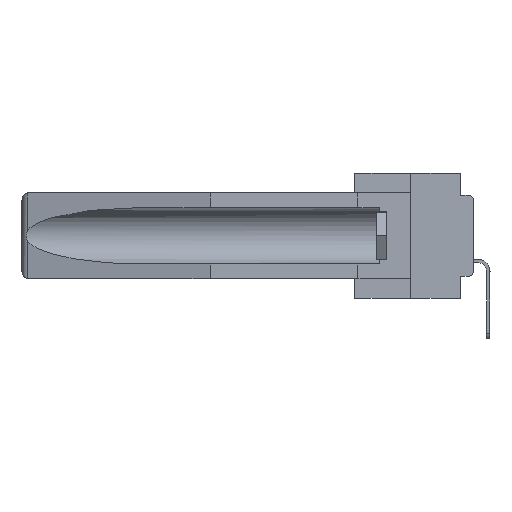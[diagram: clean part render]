
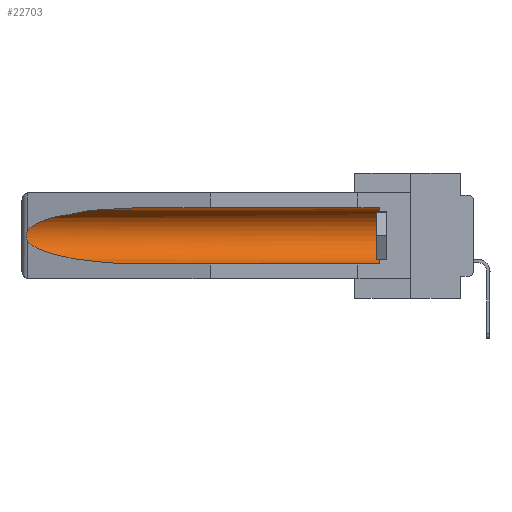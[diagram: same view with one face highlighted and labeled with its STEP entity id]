
A CAD part, left-side view. The second image highlights one B-rep face of the part: STEP entity #22703.
In plain terms, the highlighted cylindrical face has radius 2.857 mm (diameter 5.715 mm), a partial arc.
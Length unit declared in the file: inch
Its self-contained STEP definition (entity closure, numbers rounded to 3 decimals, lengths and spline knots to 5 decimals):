
#1661 = ORIENTED_EDGE ( 'NONE', *, *, #19579, .T. ) ;
#3295 = CARTESIAN_POINT ( 'NONE',  ( 0.2673, 1.5327, -0.16383 ) ) ;
#3520 = CARTESIAN_POINT ( 'NONE',  ( 0.155, 0.126, -0.059 ) ) ;
#3629 = EDGE_CURVE ( 'NONE', #25369, #14573, #30500, .T. ) ;
#4773 = EDGE_LOOP ( 'NONE', ( #11918, #1661, #10795, #9263, #9415, #20412 ) ) ;
#5623 = CARTESIAN_POINT ( 'NONE',  ( 0.26654, 1.53092, -0.15636 ) ) ;
#5877 = VECTOR ( 'NONE', #8339, 39.37008 ) ;
#6345 =( BOUNDED_CURVE ( )  B_SPLINE_CURVE ( 3, ( #18816, #21116, #14318, #19122 ),
 .UNSPECIFIED., .F., .F. ) 
 B_SPLINE_CURVE_WITH_KNOTS ( ( 4, 4 ),
 ( 0.1948, 1.5708 ),
 .UNSPECIFIED. ) 
 CURVE ( )  GEOMETRIC_REPRESENTATION_ITEM ( )  RATIONAL_B_SPLINE_CURVE ( ( 1., 0.848, 0.848, 1. ) ) 
 REPRESENTATION_ITEM ( '' )  );
#6880 = CARTESIAN_POINT ( 'NONE',  ( 0.26537, 1.52718, -0.19328 ) ) ;
#7287 = CARTESIAN_POINT ( 'NONE',  ( 0.155, 0.126, -0.1715 ) ) ;
#7567 = CARTESIAN_POINT ( 'NONE',  ( 0.155, 1.07973, -0.284 ) ) ;
#7580 = EDGE_CURVE ( 'NONE', #14573, #22712, #9837, .T. ) ;
#7781 = CARTESIAN_POINT ( 'NONE',  ( 0.2675, 1.53308, -0.17534 ) ) ;
#7938 = CARTESIAN_POINT ( 'NONE',  ( 0.26655, 1.53094, -0.18657 ) ) ;
#8052 = LINE ( 'NONE', #10712, #19145 ) ;
#8318 = CARTESIAN_POINT ( 'NONE',  ( 0.21114, 1.30732, -0.059 ) ) ;
#8339 = DIRECTION ( 'NONE',  ( 0., 1., 0. ) ) ;
#8440 = CARTESIAN_POINT ( 'NONE',  ( 0.26597, 1.52961, -0.15275 ) ) ;
#8776 = FACE_OUTER_BOUND ( 'NONE', #4773, .T. ) ;
#9240 = AXIS2_PLACEMENT_3D ( 'NONE', #21017, #23801, #31074 ) ;
#9263 = ORIENTED_EDGE ( 'NONE', *, *, #13579, .F. ) ;
#9415 = ORIENTED_EDGE ( 'NONE', *, *, #3629, .T. ) ;
#9731 =( BOUNDED_CURVE ( )  B_SPLINE_CURVE ( 3, ( #15768, #8318, #21047, #15606 ),
 .UNSPECIFIED., .F., .F. ) 
 B_SPLINE_CURVE_WITH_KNOTS ( ( 4, 4 ),
 ( 4.71239, 6.08839 ),
 .UNSPECIFIED. ) 
 CURVE ( )  GEOMETRIC_REPRESENTATION_ITEM ( )  RATIONAL_B_SPLINE_CURVE ( ( 1., 0.848, 0.848, 1. ) ) 
 REPRESENTATION_ITEM ( '' )  );
#9837 = LINE ( 'NONE', #19929, #5877 ) ;
#10291 = EDGE_CURVE ( 'NONE', #24259, #24067, #6345, .T. ) ;
#10712 = CARTESIAN_POINT ( 'NONE',  ( 0.155, -0.30754, -0.284 ) ) ;
#10795 = ORIENTED_EDGE ( 'NONE', *, *, #10291, .T. ) ;
#11918 = ORIENTED_EDGE ( 'NONE', *, *, #19132, .T. ) ;
#13579 = EDGE_CURVE ( 'NONE', #25369, #24067, #8052, .T. ) ;
#14318 = CARTESIAN_POINT ( 'NONE',  ( 0.21114, 1.30732, -0.284 ) ) ;
#14573 = VERTEX_POINT ( 'NONE', #3520 ) ;
#14882 = DIRECTION ( 'NONE',  ( 0., 0., 1. ) ) ;
#15201 = DIRECTION ( 'NONE',  ( 0., 1., 0. ) ) ;
#15606 = CARTESIAN_POINT ( 'NONE',  ( 0.26537, 1.52718, -0.14972 ) ) ;
#15768 = CARTESIAN_POINT ( 'NONE',  ( 0.155, 1.07973, -0.059 ) ) ;
#18533 = CARTESIAN_POINT ( 'NONE',  ( 0.2673, 1.53269, -0.17917 ) ) ;
#18542 = CARTESIAN_POINT ( 'NONE',  ( 0.155, 1.07973, -0.059 ) ) ;
#18816 = CARTESIAN_POINT ( 'NONE',  ( 0.26537, 1.52718, -0.19328 ) ) ;
#18875 = CYLINDRICAL_SURFACE ( 'NONE', #9240, 0.1125 ) ;
#19122 = CARTESIAN_POINT ( 'NONE',  ( 0.155, 1.07973, -0.284 ) ) ;
#19132 = EDGE_CURVE ( 'NONE', #22712, #27759, #9731, .T. ) ;
#19145 = VECTOR ( 'NONE', #15201, 39.37008 ) ;
#19579 = EDGE_CURVE ( 'NONE', #27759, #24259, #31575, .T. ) ;
#19929 = CARTESIAN_POINT ( 'NONE',  ( 0.155, -0.30754, -0.059 ) ) ;
#20354 = CARTESIAN_POINT ( 'NONE',  ( 0.26597, 1.5296, -0.19026 ) ) ;
#20412 = ORIENTED_EDGE ( 'NONE', *, *, #7580, .T. ) ;
#21017 = CARTESIAN_POINT ( 'NONE',  ( 0.155, -0.30754, -0.1715 ) ) ;
#21047 = CARTESIAN_POINT ( 'NONE',  ( 0.25451, 1.48313, -0.09465 ) ) ;
#21116 = CARTESIAN_POINT ( 'NONE',  ( 0.25451, 1.48313, -0.24835 ) ) ;
#22703 = ADVANCED_FACE ( 'NONE', ( #8776 ), #18875, .F. ) ;
#22712 = VERTEX_POINT ( 'NONE', #18542 ) ;
#22792 = DIRECTION ( 'NONE',  ( 0., -1., 0. ) ) ;
#23801 = DIRECTION ( 'NONE',  ( 0., 1., 0. ) ) ;
#24067 = VERTEX_POINT ( 'NONE', #7567 ) ;
#24259 = VERTEX_POINT ( 'NONE', #6880 ) ;
#25369 = VERTEX_POINT ( 'NONE', #28227 ) ;
#25634 = CARTESIAN_POINT ( 'NONE',  ( 0.26537, 1.52718, -0.14972 ) ) ;
#25984 = CARTESIAN_POINT ( 'NONE',  ( 0.26537, 1.52718, -0.14972 ) ) ;
#27328 = AXIS2_PLACEMENT_3D ( 'NONE', #7287, #22792, #14882 ) ;
#27759 = VERTEX_POINT ( 'NONE', #25984 ) ;
#28227 = CARTESIAN_POINT ( 'NONE',  ( 0.155, 0.126, -0.284 ) ) ;
#28586 = CARTESIAN_POINT ( 'NONE',  ( 0.26537, 1.52718, -0.19328 ) ) ;
#30500 = CIRCLE ( 'NONE', #27328, 0.1125 ) ;
#31065 = CARTESIAN_POINT ( 'NONE',  ( 0.2675, 1.53308, -0.16763 ) ) ;
#31074 = DIRECTION ( 'NONE',  ( 0., 0., 1. ) ) ;
#31575 = B_SPLINE_CURVE_WITH_KNOTS ( 'NONE', 3,
 ( #25634, #8440, #5623, #3295, #31065, #7781, #18533, #7938, #20354, #28586 ),
 .UNSPECIFIED., .F., .F.,
 ( 4, 2, 2, 2, 4 ),
 ( 0., 0.00029, 0.00058, 0.00087, 0.00117 ),
 .UNSPECIFIED. ) ;
